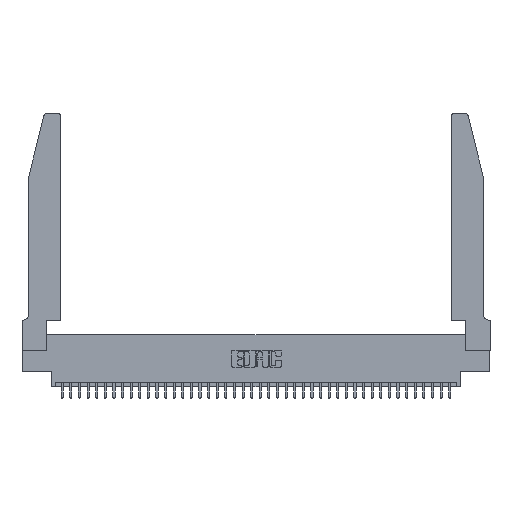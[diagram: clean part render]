
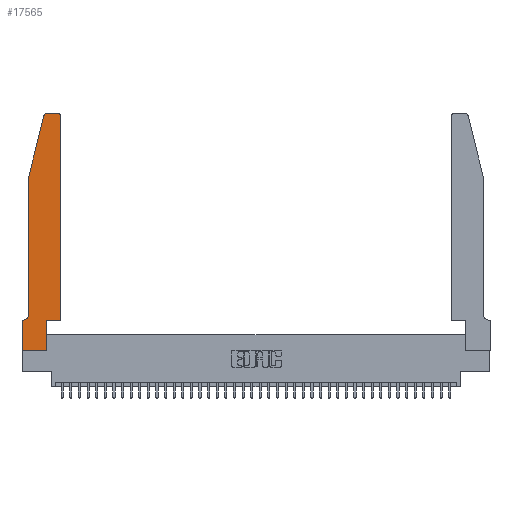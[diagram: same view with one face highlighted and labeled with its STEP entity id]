
A CAD part, top view. The second image highlights one B-rep face of the part: STEP entity #17565.
In plain terms, the highlighted planar face has unit normal (0, 0, 1).
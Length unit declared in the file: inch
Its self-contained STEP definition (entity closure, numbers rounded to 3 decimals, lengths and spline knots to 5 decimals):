
#174 = AXIS2_PLACEMENT_3D ( 'NONE', #22179, #3347, #25341 ) ;
#430 = DIRECTION ( 'NONE',  ( 0., -1., 0. ) ) ;
#985 = ORIENTED_EDGE ( 'NONE', *, *, #30490, .T. ) ;
#1059 = EDGE_CURVE ( 'NONE', #37861, #27439, #32282, .T. ) ;
#1122 = LINE ( 'NONE', #4789, #17932 ) ;
#1937 = DIRECTION ( 'NONE',  ( -1., 0., 0. ) ) ;
#2081 = EDGE_LOOP ( 'NONE', ( #4269, #9552, #22916, #34446, #17433, #11877, #11434, #985, #32074, #2862, #30826, #31912 ) ) ;
#2160 = CARTESIAN_POINT ( 'NONE',  ( 0.0055, 0.35, 0.37 ) ) ;
#2364 = DIRECTION ( 'NONE',  ( 1., 0., 0. ) ) ;
#2862 = ORIENTED_EDGE ( 'NONE', *, *, #36437, .T. ) ;
#3347 = DIRECTION ( 'NONE',  ( 0., 0., 1. ) ) ;
#3851 = CARTESIAN_POINT ( 'NONE',  ( 0.4505, 0.35, 0.37 ) ) ;
#4004 = LINE ( 'NONE', #28774, #28063 ) ;
#4269 = ORIENTED_EDGE ( 'NONE', *, *, #38827, .T. ) ;
#4296 = LINE ( 'NONE', #5031, #28321 ) ;
#4789 = CARTESIAN_POINT ( 'NONE',  ( 0.2605, 2.75, 0.37 ) ) ;
#5031 = CARTESIAN_POINT ( 'NONE',  ( 0.0755, 0.35, 0.37 ) ) ;
#5966 = VERTEX_POINT ( 'NONE', #17777 ) ;
#5995 = VECTOR ( 'NONE', #39479, 39.37008 ) ;
#6186 = DIRECTION ( 'NONE',  ( 0., 0., -1. ) ) ;
#7044 = VERTEX_POINT ( 'NONE', #33728 ) ;
#7986 = EDGE_CURVE ( 'NONE', #21181, #35906, #29553, .T. ) ;
#8533 = AXIS2_PLACEMENT_3D ( 'NONE', #38267, #13611, #35327 ) ;
#8664 = EDGE_CURVE ( 'NONE', #8842, #26650, #4004, .T. ) ;
#8842 = VERTEX_POINT ( 'NONE', #23323 ) ;
#9552 = ORIENTED_EDGE ( 'NONE', *, *, #7986, .T. ) ;
#9947 = CARTESIAN_POINT ( 'NONE',  ( 0., 0., 0.37 ) ) ;
#11236 = EDGE_CURVE ( 'NONE', #16648, #18404, #4296, .T. ) ;
#11311 = AXIS2_PLACEMENT_3D ( 'NONE', #31766, #13161, #34889 ) ;
#11434 = ORIENTED_EDGE ( 'NONE', *, *, #19685, .T. ) ;
#11877 = ORIENTED_EDGE ( 'NONE', *, *, #11236, .T. ) ;
#13161 = DIRECTION ( 'NONE',  ( 0., 0., 1. ) ) ;
#13611 = DIRECTION ( 'NONE',  ( 0., 0., 1. ) ) ;
#14275 = EDGE_CURVE ( 'NONE', #7044, #31273, #26215, .T. ) ;
#14349 = VECTOR ( 'NONE', #15802, 39.37008 ) ;
#15262 = CARTESIAN_POINT ( 'NONE',  ( 0.284, 2.75, 0.37 ) ) ;
#15802 = DIRECTION ( 'NONE',  ( -0.239, -0.971, 0. ) ) ;
#15972 = VERTEX_POINT ( 'NONE', #3851 ) ;
#16331 = CARTESIAN_POINT ( 'NONE',  ( 0.2865, 0.35, 0.37 ) ) ;
#16648 = VERTEX_POINT ( 'NONE', #2160 ) ;
#17158 = DIRECTION ( 'NONE',  ( 0., 1., 0. ) ) ;
#17433 = ORIENTED_EDGE ( 'NONE', *, *, #31238, .T. ) ;
#17565 = ADVANCED_FACE ( 'NONE', ( #29625 ), #26053, .T. ) ;
#17777 = CARTESIAN_POINT ( 'NONE',  ( 0., 0., 0.37 ) ) ;
#17932 = VECTOR ( 'NONE', #23587, 39.37008 ) ;
#18404 = VERTEX_POINT ( 'NONE', #20487 ) ;
#19238 = CARTESIAN_POINT ( 'NONE',  ( 0.0755, 0.42, 0.37 ) ) ;
#19685 = EDGE_CURVE ( 'NONE', #18404, #5966, #31432, .T. ) ;
#20487 = CARTESIAN_POINT ( 'NONE',  ( 0., 0.35, 0.37 ) ) ;
#20513 = LINE ( 'NONE', #21222, #29783 ) ;
#21181 = VERTEX_POINT ( 'NONE', #15262 ) ;
#21222 = CARTESIAN_POINT ( 'NONE',  ( 0.4505, 0.35, 0.37 ) ) ;
#21775 = EDGE_CURVE ( 'NONE', #15972, #37861, #35574, .T. ) ;
#22111 = CARTESIAN_POINT ( 'NONE',  ( 0.0755, 2., 0.37 ) ) ;
#22179 = CARTESIAN_POINT ( 'NONE',  ( 0.4205, 2.72, 0.37 ) ) ;
#22667 = LINE ( 'NONE', #27142, #5995 ) ;
#22916 = ORIENTED_EDGE ( 'NONE', *, *, #26610, .T. ) ;
#23323 = CARTESIAN_POINT ( 'NONE',  ( 0.0755, 2., 0.37 ) ) ;
#23587 = DIRECTION ( 'NONE',  ( -1., 0., 0. ) ) ;
#24985 = CARTESIAN_POINT ( 'NONE',  ( 0.0055, 0.42, 0.37 ) ) ;
#25341 = DIRECTION ( 'NONE',  ( 1., 0., 0. ) ) ;
#26053 = PLANE ( 'NONE',  #8533 ) ;
#26079 = AXIS2_PLACEMENT_3D ( 'NONE', #24985, #6186, #28102 ) ;
#26215 = LINE ( 'NONE', #35899, #35360 ) ;
#26610 = EDGE_CURVE ( 'NONE', #35906, #8842, #37154, .T. ) ;
#26650 = VERTEX_POINT ( 'NONE', #19238 ) ;
#27142 = CARTESIAN_POINT ( 'NONE',  ( 0., 0., 0.37 ) ) ;
#27395 = VECTOR ( 'NONE', #39346, 39.37008 ) ;
#27439 = VERTEX_POINT ( 'NONE', #29102 ) ;
#28031 = CARTESIAN_POINT ( 'NONE',  ( 0.4505, 2.72, 0.37 ) ) ;
#28063 = VECTOR ( 'NONE', #430, 39.37008 ) ;
#28102 = DIRECTION ( 'NONE',  ( -1., 0., 0. ) ) ;
#28321 = VECTOR ( 'NONE', #1937, 39.37008 ) ;
#28463 = CIRCLE ( 'NONE', #26079, 0.07 ) ;
#28620 = DIRECTION ( 'NONE',  ( 0., -1., 0. ) ) ;
#28774 = CARTESIAN_POINT ( 'NONE',  ( 0.0755, 2., 0.37 ) ) ;
#29102 = CARTESIAN_POINT ( 'NONE',  ( 0.4205, 2.75, 0.37 ) ) ;
#29553 = CIRCLE ( 'NONE', #11311, 0.03 ) ;
#29625 = FACE_OUTER_BOUND ( 'NONE', #2081, .T. ) ;
#29783 = VECTOR ( 'NONE', #2364, 39.37008 ) ;
#30087 = CARTESIAN_POINT ( 'NONE',  ( 0.4505, 0.35, 0.37 ) ) ;
#30490 = EDGE_CURVE ( 'NONE', #5966, #7044, #22667, .T. ) ;
#30826 = ORIENTED_EDGE ( 'NONE', *, *, #21775, .T. ) ;
#31238 = EDGE_CURVE ( 'NONE', #26650, #16648, #28463, .T. ) ;
#31273 = VERTEX_POINT ( 'NONE', #16331 ) ;
#31432 = LINE ( 'NONE', #9947, #39604 ) ;
#31766 = CARTESIAN_POINT ( 'NONE',  ( 0.284, 2.72, 0.37 ) ) ;
#31912 = ORIENTED_EDGE ( 'NONE', *, *, #1059, .T. ) ;
#32074 = ORIENTED_EDGE ( 'NONE', *, *, #14275, .T. ) ;
#32282 = CIRCLE ( 'NONE', #174, 0.03 ) ;
#33728 = CARTESIAN_POINT ( 'NONE',  ( 0.2865, 0., 0.37 ) ) ;
#33995 = CARTESIAN_POINT ( 'NONE',  ( 0.25487, 2.72718, 0.37 ) ) ;
#34446 = ORIENTED_EDGE ( 'NONE', *, *, #8664, .T. ) ;
#34889 = DIRECTION ( 'NONE',  ( 1., 0., 0. ) ) ;
#35327 = DIRECTION ( 'NONE',  ( 1., 0., 0. ) ) ;
#35360 = VECTOR ( 'NONE', #17158, 39.37008 ) ;
#35574 = LINE ( 'NONE', #30087, #27395 ) ;
#35899 = CARTESIAN_POINT ( 'NONE',  ( 0.2865, 0.35, 0.37 ) ) ;
#35906 = VERTEX_POINT ( 'NONE', #33995 ) ;
#36437 = EDGE_CURVE ( 'NONE', #31273, #15972, #20513, .T. ) ;
#37154 = LINE ( 'NONE', #22111, #14349 ) ;
#37861 = VERTEX_POINT ( 'NONE', #28031 ) ;
#38267 = CARTESIAN_POINT ( 'NONE',  ( 0., 0.35, 0.37 ) ) ;
#38827 = EDGE_CURVE ( 'NONE', #27439, #21181, #1122, .T. ) ;
#39346 = DIRECTION ( 'NONE',  ( 0., 1., 0. ) ) ;
#39479 = DIRECTION ( 'NONE',  ( 1., 0., 0. ) ) ;
#39604 = VECTOR ( 'NONE', #28620, 39.37008 ) ;
